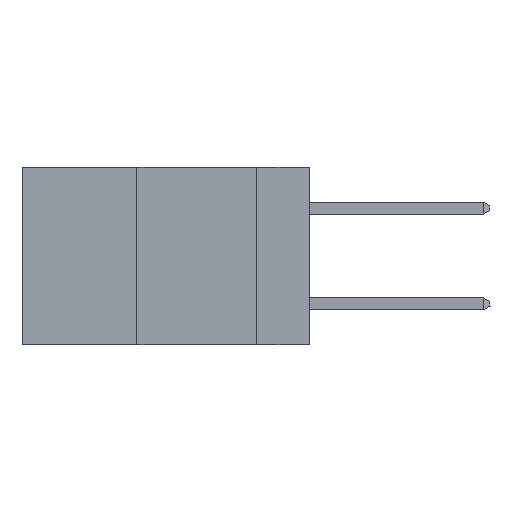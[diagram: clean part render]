
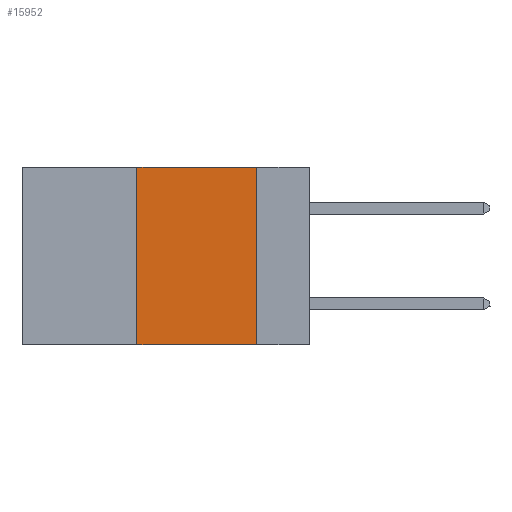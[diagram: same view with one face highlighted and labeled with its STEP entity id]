
A CAD part, left-side view. The second image highlights one B-rep face of the part: STEP entity #15952.
In plain terms, the highlighted planar face has unit normal (-1, 0, 0).
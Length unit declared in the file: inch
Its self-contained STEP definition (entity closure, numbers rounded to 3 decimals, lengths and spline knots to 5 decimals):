
#786 = EDGE_CURVE ( 'NONE', #2121, #1361, #9676, .T. ) ;
#1361 = VERTEX_POINT ( 'NONE', #11047 ) ;
#2121 = VERTEX_POINT ( 'NONE', #4095 ) ;
#2468 = CARTESIAN_POINT ( 'NONE',  ( 0., 0.11, 0. ) ) ;
#2575 = EDGE_CURVE ( 'NONE', #2121, #15088, #11395, .T. ) ;
#2585 = CARTESIAN_POINT ( 'NONE',  ( 0., 0.11, -0.37 ) ) ;
#3410 = ORIENTED_EDGE ( 'NONE', *, *, #2575, .T. ) ;
#3473 = CARTESIAN_POINT ( 'NONE',  ( 0., 0.6, -0.37 ) ) ;
#4095 = CARTESIAN_POINT ( 'NONE',  ( 0., 0.36, -0.37 ) ) ;
#4768 = CARTESIAN_POINT ( 'NONE',  ( 0., 0.11, 0. ) ) ;
#4816 = FACE_OUTER_BOUND ( 'NONE', #6461, .T. ) ;
#5389 = EDGE_CURVE ( 'NONE', #6768, #15088, #12815, .T. ) ;
#5638 = AXIS2_PLACEMENT_3D ( 'NONE', #7143, #8485, #14731 ) ;
#5682 = DIRECTION ( 'NONE',  ( 0., -1., 0. ) ) ;
#6461 = EDGE_LOOP ( 'NONE', ( #14878, #16129, #10186, #3410 ) ) ;
#6768 = VERTEX_POINT ( 'NONE', #2468 ) ;
#7143 = CARTESIAN_POINT ( 'NONE',  ( 0., 0.6, 0. ) ) ;
#8052 = VECTOR ( 'NONE', #5682, 39.37008 ) ;
#8376 = PLANE ( 'NONE',  #5638 ) ;
#8485 = DIRECTION ( 'NONE',  ( 1., 0., 0. ) ) ;
#9491 = VECTOR ( 'NONE', #9824, 39.37008 ) ;
#9510 = DIRECTION ( 'NONE',  ( 0., 0., 1. ) ) ;
#9676 = LINE ( 'NONE', #9734, #13394 ) ;
#9734 = CARTESIAN_POINT ( 'NONE',  ( 0., 0.36, 0. ) ) ;
#9824 = DIRECTION ( 'NONE',  ( 0., 0., -1. ) ) ;
#10186 = ORIENTED_EDGE ( 'NONE', *, *, #786, .F. ) ;
#10444 = EDGE_CURVE ( 'NONE', #1361, #6768, #13558, .T. ) ;
#10960 = DIRECTION ( 'NONE',  ( 0., -1., 0. ) ) ;
#11047 = CARTESIAN_POINT ( 'NONE',  ( 0., 0.36, 0. ) ) ;
#11395 = LINE ( 'NONE', #3473, #14598 ) ;
#11880 = CARTESIAN_POINT ( 'NONE',  ( 0., 0.6, 0. ) ) ;
#12815 = LINE ( 'NONE', #4768, #9491 ) ;
#13394 = VECTOR ( 'NONE', #9510, 39.37008 ) ;
#13558 = LINE ( 'NONE', #11880, #8052 ) ;
#14598 = VECTOR ( 'NONE', #10960, 39.37008 ) ;
#14731 = DIRECTION ( 'NONE',  ( 0., 0., -1. ) ) ;
#14878 = ORIENTED_EDGE ( 'NONE', *, *, #5389, .F. ) ;
#15088 = VERTEX_POINT ( 'NONE', #2585 ) ;
#15952 = ADVANCED_FACE ( 'NONE', ( #4816 ), #8376, .F. ) ;
#16129 = ORIENTED_EDGE ( 'NONE', *, *, #10444, .F. ) ;
